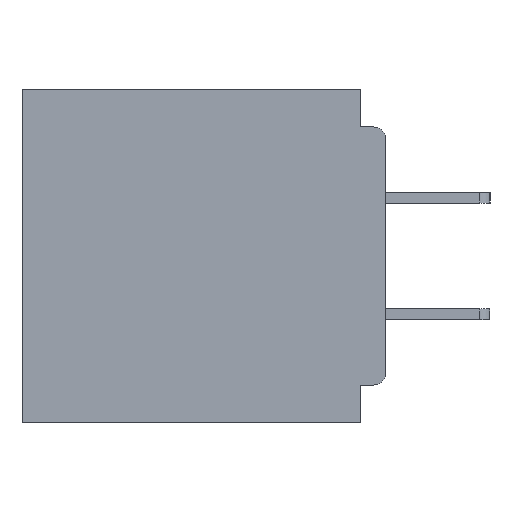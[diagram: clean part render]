
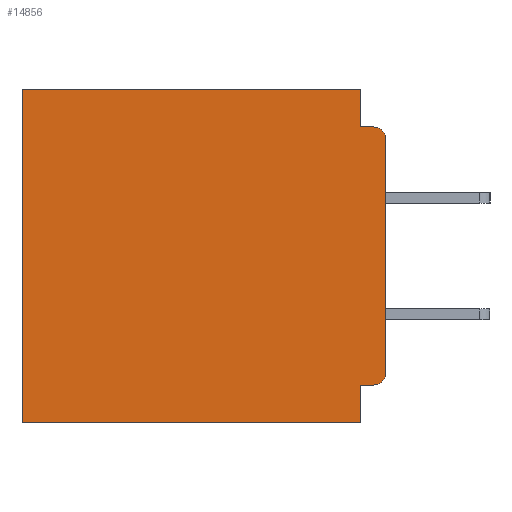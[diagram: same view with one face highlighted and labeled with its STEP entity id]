
A CAD part, left-side view. The second image highlights one B-rep face of the part: STEP entity #14856.
In plain terms, the highlighted planar face has unit normal (-1, 0, 0).
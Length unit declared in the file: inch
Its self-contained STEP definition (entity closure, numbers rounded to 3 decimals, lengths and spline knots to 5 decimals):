
#703 = AXIS2_PLACEMENT_3D ( 'NONE', #36647, #883, #21889 ) ;
#768 = VECTOR ( 'NONE', #4998, 39.37008 ) ;
#883 = DIRECTION ( 'NONE',  ( 1., 0., 0. ) ) ;
#2205 = VERTEX_POINT ( 'NONE', #3688 ) ;
#2357 = VECTOR ( 'NONE', #20316, 39.37008 ) ;
#2692 = CARTESIAN_POINT ( 'NONE',  ( 0.3, 0., -0.355 ) ) ;
#3688 = CARTESIAN_POINT ( 'NONE',  ( 0.3, 0.437, -0.4 ) ) ;
#4115 = ORIENTED_EDGE ( 'NONE', *, *, #14777, .F. ) ;
#4998 = DIRECTION ( 'NONE',  ( 0., 1., 0. ) ) ;
#5279 = VERTEX_POINT ( 'NONE', #28002 ) ;
#5353 = CARTESIAN_POINT ( 'NONE',  ( 0.3, 0., -0.4 ) ) ;
#5380 = VECTOR ( 'NONE', #22565, 39.37008 ) ;
#6100 = DIRECTION ( 'NONE',  ( -1., 0., 0. ) ) ;
#6355 = ORIENTED_EDGE ( 'NONE', *, *, #33992, .F. ) ;
#6502 = VERTEX_POINT ( 'NONE', #24911 ) ;
#6573 = LINE ( 'NONE', #15766, #37370 ) ;
#6622 = AXIS2_PLACEMENT_3D ( 'NONE', #24140, #6100, #27104 ) ;
#6633 = AXIS2_PLACEMENT_3D ( 'NONE', #35350, #17471, #38311 ) ;
#6860 = EDGE_CURVE ( 'NONE', #24176, #17993, #15773, .T. ) ;
#6931 = ORIENTED_EDGE ( 'NONE', *, *, #15811, .F. ) ;
#8972 = CARTESIAN_POINT ( 'NONE',  ( 0.3, 0.031, -0.4 ) ) ;
#9383 = VERTEX_POINT ( 'NONE', #15860 ) ;
#10257 = EDGE_CURVE ( 'NONE', #36458, #9383, #33070, .T. ) ;
#11302 = ORIENTED_EDGE ( 'NONE', *, *, #6860, .F. ) ;
#11377 = VECTOR ( 'NONE', #14078, 39.37008 ) ;
#12011 = CARTESIAN_POINT ( 'NONE',  ( 0.3, 0.031, -0.045 ) ) ;
#12314 = CARTESIAN_POINT ( 'NONE',  ( 0.3, 0., -0.045 ) ) ;
#12826 = PLANE ( 'NONE',  #703 ) ;
#13036 = FACE_OUTER_BOUND ( 'NONE', #13479, .T. ) ;
#13479 = EDGE_LOOP ( 'NONE', ( #21992, #28040, #4115, #6355, #26044, #35781, #21384, #6931, #11302, #16096 ) ) ;
#14078 = DIRECTION ( 'NONE',  ( 0., 1., 0. ) ) ;
#14658 = CARTESIAN_POINT ( 'NONE',  ( 0.3, 0., -0.06 ) ) ;
#14777 = EDGE_CURVE ( 'NONE', #35366, #9383, #22910, .T. ) ;
#14856 = ADVANCED_FACE ( 'NONE', ( #13036 ), #12826, .F. ) ;
#14899 = VECTOR ( 'NONE', #33326, 39.37008 ) ;
#15766 = CARTESIAN_POINT ( 'NONE',  ( 0.3, 0.437, -0.4 ) ) ;
#15773 = LINE ( 'NONE', #2692, #768 ) ;
#15811 = EDGE_CURVE ( 'NONE', #17993, #18759, #33978, .T. ) ;
#15860 = CARTESIAN_POINT ( 'NONE',  ( 0.3, 0.015, -0.045 ) ) ;
#15988 = CARTESIAN_POINT ( 'NONE',  ( 0.3, 0.031, -0.355 ) ) ;
#16096 = ORIENTED_EDGE ( 'NONE', *, *, #20526, .T. ) ;
#17423 = CARTESIAN_POINT ( 'NONE',  ( 0.3, 0.031, 0. ) ) ;
#17471 = DIRECTION ( 'NONE',  ( -1., 0., 0. ) ) ;
#17993 = VERTEX_POINT ( 'NONE', #15988 ) ;
#18759 = VERTEX_POINT ( 'NONE', #34590 ) ;
#19258 = EDGE_CURVE ( 'NONE', #26096, #2205, #6573, .T. ) ;
#19322 = LINE ( 'NONE', #20118, #11377 ) ;
#19557 = CARTESIAN_POINT ( 'NONE',  ( 0.3, 0.437, 0. ) ) ;
#19851 = EDGE_CURVE ( 'NONE', #18759, #2205, #25389, .T. ) ;
#20118 = CARTESIAN_POINT ( 'NONE',  ( 0.3, 0., 0. ) ) ;
#20316 = DIRECTION ( 'NONE',  ( 0., 1., 0. ) ) ;
#20526 = EDGE_CURVE ( 'NONE', #24176, #6502, #38274, .T. ) ;
#21384 = ORIENTED_EDGE ( 'NONE', *, *, #19851, .F. ) ;
#21889 = DIRECTION ( 'NONE',  ( 0., 0., -1. ) ) ;
#21992 = ORIENTED_EDGE ( 'NONE', *, *, #34472, .F. ) ;
#22349 = LINE ( 'NONE', #17423, #29320 ) ;
#22565 = DIRECTION ( 'NONE',  ( 0., 0., -1. ) ) ;
#22910 = LINE ( 'NONE', #12314, #14899 ) ;
#23960 = DIRECTION ( 'NONE',  ( 0., 0., -1. ) ) ;
#24140 = CARTESIAN_POINT ( 'NONE',  ( 0.3, 0.015, -0.34 ) ) ;
#24176 = VERTEX_POINT ( 'NONE', #37928 ) ;
#24911 = CARTESIAN_POINT ( 'NONE',  ( 0.3, 0., -0.34 ) ) ;
#25389 = LINE ( 'NONE', #5353, #2357 ) ;
#25599 = CARTESIAN_POINT ( 'NONE',  ( 0.3, 0., -0.4 ) ) ;
#25627 = EDGE_CURVE ( 'NONE', #5279, #26096, #19322, .T. ) ;
#26044 = ORIENTED_EDGE ( 'NONE', *, *, #25627, .T. ) ;
#26096 = VERTEX_POINT ( 'NONE', #19557 ) ;
#27104 = DIRECTION ( 'NONE',  ( 0., 0., -1. ) ) ;
#27830 = DIRECTION ( 'NONE',  ( 0., 0., -1. ) ) ;
#28002 = CARTESIAN_POINT ( 'NONE',  ( 0.3, 0.031, 0. ) ) ;
#28040 = ORIENTED_EDGE ( 'NONE', *, *, #10257, .T. ) ;
#29283 = LINE ( 'NONE', #25599, #5380 ) ;
#29320 = VECTOR ( 'NONE', #29361, 39.37008 ) ;
#29361 = DIRECTION ( 'NONE',  ( 0., 0., -1. ) ) ;
#33042 = VECTOR ( 'NONE', #23960, 39.37008 ) ;
#33070 = CIRCLE ( 'NONE', #6633, 0.015 ) ;
#33326 = DIRECTION ( 'NONE',  ( 0., -1., 0. ) ) ;
#33978 = LINE ( 'NONE', #8972, #33042 ) ;
#33992 = EDGE_CURVE ( 'NONE', #5279, #35366, #22349, .T. ) ;
#34472 = EDGE_CURVE ( 'NONE', #36458, #6502, #29283, .T. ) ;
#34590 = CARTESIAN_POINT ( 'NONE',  ( 0.3, 0.031, -0.4 ) ) ;
#35350 = CARTESIAN_POINT ( 'NONE',  ( 0.3, 0.015, -0.06 ) ) ;
#35366 = VERTEX_POINT ( 'NONE', #12011 ) ;
#35781 = ORIENTED_EDGE ( 'NONE', *, *, #19258, .T. ) ;
#36458 = VERTEX_POINT ( 'NONE', #14658 ) ;
#36647 = CARTESIAN_POINT ( 'NONE',  ( 0.3, 0., -0.4 ) ) ;
#37370 = VECTOR ( 'NONE', #27830, 39.37008 ) ;
#37928 = CARTESIAN_POINT ( 'NONE',  ( 0.3, 0.015, -0.355 ) ) ;
#38274 = CIRCLE ( 'NONE', #6622, 0.015 ) ;
#38311 = DIRECTION ( 'NONE',  ( 0., 0., -1. ) ) ;
